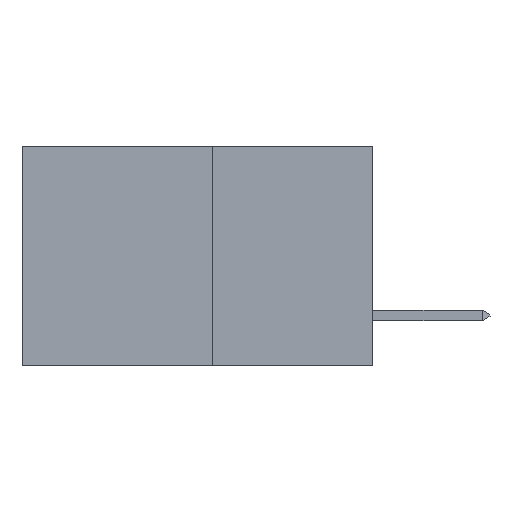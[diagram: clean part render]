
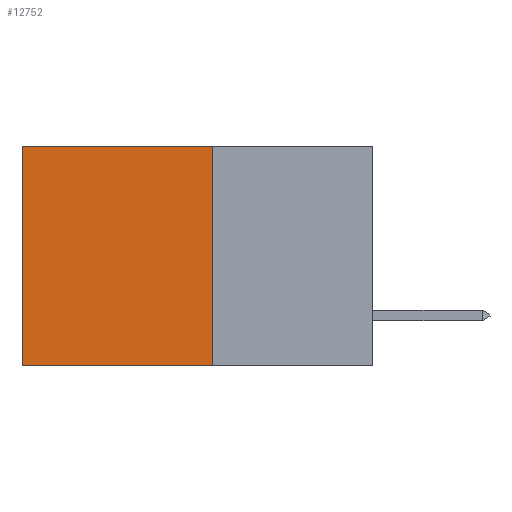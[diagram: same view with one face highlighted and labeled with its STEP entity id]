
A CAD part, left-side view. The second image highlights one B-rep face of the part: STEP entity #12752.
In plain terms, the highlighted planar face has unit normal (-1, 0, 0).
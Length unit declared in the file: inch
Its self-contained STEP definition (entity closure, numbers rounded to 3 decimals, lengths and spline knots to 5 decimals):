
#41 = CARTESIAN_POINT ( 'NONE',  ( 0.277, 0.27, 0. ) ) ;
#52 = ORIENTED_EDGE ( 'NONE', *, *, #10480, .T. ) ;
#1059 = DIRECTION ( 'NONE',  ( 0., 1., 0. ) ) ;
#1106 = VECTOR ( 'NONE', #7011, 39.37008 ) ;
#1327 = DIRECTION ( 'NONE',  ( 1., 0., 0. ) ) ;
#1360 = ORIENTED_EDGE ( 'NONE', *, *, #6140, .F. ) ;
#1382 = CARTESIAN_POINT ( 'NONE',  ( 0.277, 0.59, 0. ) ) ;
#1724 = VERTEX_POINT ( 'NONE', #1382 ) ;
#1770 = LINE ( 'NONE', #11989, #1106 ) ;
#1989 = EDGE_CURVE ( 'NONE', #9652, #6488, #9286, .T. ) ;
#2096 = EDGE_LOOP ( 'NONE', ( #52, #1360, #4030, #6173 ) ) ;
#3238 = DIRECTION ( 'NONE',  ( 0., 0., -1. ) ) ;
#4030 = ORIENTED_EDGE ( 'NONE', *, *, #1989, .F. ) ;
#5535 = VECTOR ( 'NONE', #1059, 39.37008 ) ;
#5868 = LINE ( 'NONE', #41, #5535 ) ;
#6070 = CARTESIAN_POINT ( 'NONE',  ( 0.277, 0.27, 0. ) ) ;
#6140 = EDGE_CURVE ( 'NONE', #6488, #11703, #1770, .T. ) ;
#6173 = ORIENTED_EDGE ( 'NONE', *, *, #10457, .T. ) ;
#6488 = VERTEX_POINT ( 'NONE', #11481 ) ;
#6605 = VECTOR ( 'NONE', #3238, 39.37008 ) ;
#6939 = CARTESIAN_POINT ( 'NONE',  ( 0.277, 0.27, -0.37 ) ) ;
#7011 = DIRECTION ( 'NONE',  ( 0., 1., 0. ) ) ;
#7422 = FACE_OUTER_BOUND ( 'NONE', #2096, .T. ) ;
#7528 = CARTESIAN_POINT ( 'NONE',  ( 0.277, 0.59, -0.37 ) ) ;
#8388 = DIRECTION ( 'NONE',  ( 0., 0., -1. ) ) ;
#8610 = DIRECTION ( 'NONE',  ( 0., 0., -1. ) ) ;
#9286 = LINE ( 'NONE', #6939, #6605 ) ;
#9652 = VERTEX_POINT ( 'NONE', #6070 ) ;
#10457 = EDGE_CURVE ( 'NONE', #9652, #1724, #5868, .T. ) ;
#10480 = EDGE_CURVE ( 'NONE', #1724, #11703, #10646, .T. ) ;
#10646 = LINE ( 'NONE', #11381, #12916 ) ;
#11185 = AXIS2_PLACEMENT_3D ( 'NONE', #12549, #1327, #8610 ) ;
#11381 = CARTESIAN_POINT ( 'NONE',  ( 0.277, 0.59, -0.37 ) ) ;
#11481 = CARTESIAN_POINT ( 'NONE',  ( 0.277, 0.27, -0.37 ) ) ;
#11586 = PLANE ( 'NONE',  #11185 ) ;
#11703 = VERTEX_POINT ( 'NONE', #7528 ) ;
#11989 = CARTESIAN_POINT ( 'NONE',  ( 0.277, 0.27, -0.37 ) ) ;
#12549 = CARTESIAN_POINT ( 'NONE',  ( 0.277, 0.27, -0.37 ) ) ;
#12752 = ADVANCED_FACE ( 'NONE', ( #7422 ), #11586, .F. ) ;
#12916 = VECTOR ( 'NONE', #8388, 39.37008 ) ;
